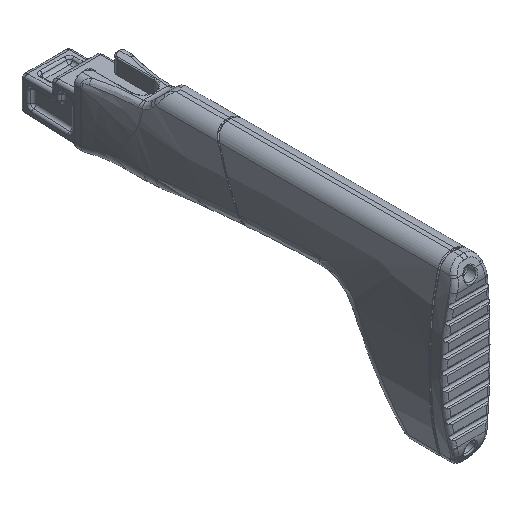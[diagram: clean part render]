
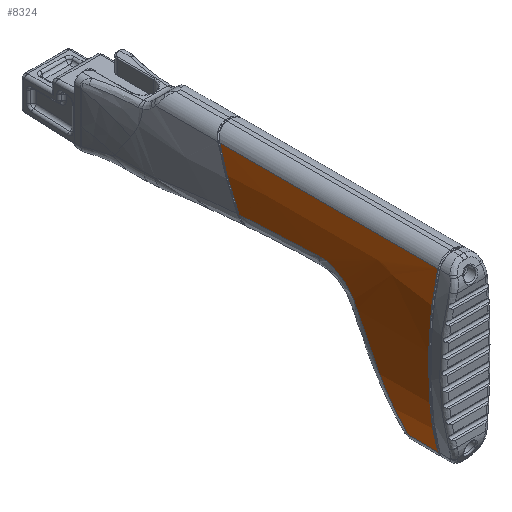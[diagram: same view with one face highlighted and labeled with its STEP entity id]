
A CAD part, isometric view. The second image highlights one B-rep face of the part: STEP entity #8324.
In plain terms, the highlighted free-form (B-spline) face has degree [1, 2] with [2, 5] control points.
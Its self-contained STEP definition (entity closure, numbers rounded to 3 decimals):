
#124=(
BOUNDED_SURFACE()
B_SPLINE_SURFACE(1,2,((#15214,#15215,#15216,#15217,#15218),(#15219,#15220,
#15221,#15222,#15223)),.UNSPECIFIED.,.F.,.F.,.F.)
B_SPLINE_SURFACE_WITH_KNOTS((2,2),(3,2,3),(0.041,2.203),
(-2.476,-1.571,-0.665),.UNSPECIFIED.)
GEOMETRIC_REPRESENTATION_ITEM()
RATIONAL_B_SPLINE_SURFACE(((1.,0.899,1.,0.899,1.),
(1.,0.899,1.,0.899,1.)))
REPRESENTATION_ITEM('')
SURFACE()
);
#330=LINE('',#15212,#699);
#331=LINE('',#15245,#700);
#699=VECTOR('',#9850,10.);
#700=VECTOR('',#9853,10.);
#1283=FACE_OUTER_BOUND('',#1867,.T.);
#1867=EDGE_LOOP('',(#5753,#5754,#5755,#5756,#5757,#5758,#5759,#5760));
#2472=B_SPLINE_CURVE_WITH_KNOTS('',3,(#14835,#14836,#14837,#14838,#14839),
 .UNSPECIFIED.,.F.,.F.,(4,1,4),(1.921,2.158,2.473),
 .UNSPECIFIED.);
#2494=B_SPLINE_CURVE_WITH_KNOTS('',3,(#15196,#15197,#15198,#15199),
 .UNSPECIFIED.,.F.,.F.,(4,4),(-0.016,0.),
 .UNSPECIFIED.);
#2495=B_SPLINE_CURVE_WITH_KNOTS('',3,(#15225,#15226,#15227,#15228),
 .UNSPECIFIED.,.F.,.F.,(4,4),(-10.9,-5.584),
 .UNSPECIFIED.);
#2496=B_SPLINE_CURVE_WITH_KNOTS('',3,(#15230,#15231,#15232,#15233,#15234,
#15235),.UNSPECIFIED.,.F.,.F.,(4,1,1,4),(-3.312,-2.366,
-1.419,0.),.UNSPECIFIED.);
#2497=B_SPLINE_CURVE_WITH_KNOTS('',3,(#15237,#15238,#15239,#15240,#15241,
#15242,#15243),.UNSPECIFIED.,.F.,.F.,(4,1,1,1,4),(-6.528,-5.596,
-4.663,-2.798,0.),.UNSPECIFIED.);
#2498=B_SPLINE_CURVE_WITH_KNOTS('',3,(#15246,#15247,#15248,#15249,#15250,
#15251,#15252,#15253,#15254,#15255,#15256),.UNSPECIFIED.,.F.,.F.,(4,1,1,
1,1,1,1,1,4),(0.,0.763,1.525,3.05,4.575,
7.626,9.151,9.913,10.676),
 .UNSPECIFIED.);
#3386=VERTEX_POINT('',#14824);
#3389=VERTEX_POINT('',#14833);
#3410=VERTEX_POINT('',#15132);
#3417=VERTEX_POINT('',#15211);
#3418=VERTEX_POINT('',#15224);
#3419=VERTEX_POINT('',#15229);
#3420=VERTEX_POINT('',#15236);
#3421=VERTEX_POINT('',#15244);
#4228=EDGE_CURVE('',#3389,#3386,#2472,.T.);
#4266=EDGE_CURVE('',#3410,#3389,#2494,.T.);
#4272=EDGE_CURVE('',#3417,#3386,#330,.T.);
#4274=EDGE_CURVE('',#3418,#3410,#2495,.T.);
#4275=EDGE_CURVE('',#3419,#3418,#2496,.T.);
#4276=EDGE_CURVE('',#3420,#3419,#2497,.T.);
#4277=EDGE_CURVE('',#3420,#3421,#331,.T.);
#4278=EDGE_CURVE('',#3417,#3421,#2498,.T.);
#5753=ORIENTED_EDGE('',*,*,#4228,.F.);
#5754=ORIENTED_EDGE('',*,*,#4266,.F.);
#5755=ORIENTED_EDGE('',*,*,#4274,.F.);
#5756=ORIENTED_EDGE('',*,*,#4275,.F.);
#5757=ORIENTED_EDGE('',*,*,#4276,.F.);
#5758=ORIENTED_EDGE('',*,*,#4277,.T.);
#5759=ORIENTED_EDGE('',*,*,#4278,.F.);
#5760=ORIENTED_EDGE('',*,*,#4272,.T.);
#8324=ADVANCED_FACE('',(#1283),#124,.T.);
#9850=DIRECTION('',(0.,1.,0.));
#9853=DIRECTION('',(0.,-1.,0.));
#14824=CARTESIAN_POINT('',(-10.031,-549.225,133.253));
#14833=CARTESIAN_POINT('',(-15.247,-567.251,103.588));
#14835=CARTESIAN_POINT('Ctrl Pts',(-15.247,-567.251,
103.588));
#14836=CARTESIAN_POINT('Ctrl Pts',(-14.803,-564.228,
108.564));
#14837=CARTESIAN_POINT('Ctrl Pts',(-13.437,-557.479,
119.672));
#14838=CARTESIAN_POINT('Ctrl Pts',(-11.378,-551.886,128.876));
#14839=CARTESIAN_POINT('Ctrl Pts',(-10.031,-549.225,
133.253));
#15132=CARTESIAN_POINT('',(-15.259,-567.335,103.451));
#15196=CARTESIAN_POINT('Ctrl Pts',(-15.259,-567.335,
103.451));
#15197=CARTESIAN_POINT('Ctrl Pts',(-15.255,-567.307,103.497));
#15198=CARTESIAN_POINT('Ctrl Pts',(-15.251,-567.279,
103.542));
#15199=CARTESIAN_POINT('Ctrl Pts',(-15.247,-567.251,
103.588));
#15211=CARTESIAN_POINT('',(-10.031,-694.735,133.253));
#15212=CARTESIAN_POINT('',(-10.031,-697.501,133.253));
#15214=CARTESIAN_POINT('Ctrl Pts',(-10.031,-694.735,133.253));
#15215=CARTESIAN_POINT('Ctrl Pts',(-16.25,-694.735,
113.043));
#15216=CARTESIAN_POINT('Ctrl Pts',(-16.25,-694.735,
80.303));
#15217=CARTESIAN_POINT('Ctrl Pts',(-16.25,-694.735,
47.563));
#15218=CARTESIAN_POINT('Ctrl Pts',(-10.031,-694.735,27.353));
#15219=CARTESIAN_POINT('Ctrl Pts',(-10.031,-549.225,133.253));
#15220=CARTESIAN_POINT('Ctrl Pts',(-16.25,-549.225,
113.043));
#15221=CARTESIAN_POINT('Ctrl Pts',(-16.25,-549.225,
80.303));
#15222=CARTESIAN_POINT('Ctrl Pts',(-16.25,-549.225,
47.563));
#15223=CARTESIAN_POINT('Ctrl Pts',(-10.031,-549.225,27.353));
#15224=CARTESIAN_POINT('',(-15.023,-620.438,105.958));
#15225=CARTESIAN_POINT('Ctrl Pts',(-15.023,-620.438,
105.958));
#15226=CARTESIAN_POINT('Ctrl Pts',(-15.051,-602.718,
105.683));
#15227=CARTESIAN_POINT('Ctrl Pts',(-15.135,-585.006,
104.846));
#15228=CARTESIAN_POINT('Ctrl Pts',(-15.259,-567.335,
103.451));
#15229=CARTESIAN_POINT('',(-16.12,-647.054,88.811));
#15230=CARTESIAN_POINT('Ctrl Pts',(-16.12,-647.054,
88.811));
#15231=CARTESIAN_POINT('Ctrl Pts',(-16.029,-645.699,
91.755));
#15232=CARTESIAN_POINT('Ctrl Pts',(-15.766,-642.052,97.18));
#15233=CARTESIAN_POINT('Ctrl Pts',(-15.225,-633.073,
104.094));
#15234=CARTESIAN_POINT('Ctrl Pts',(-15.016,-625.169,106.031));
#15235=CARTESIAN_POINT('Ctrl Pts',(-15.023,-620.438,
105.958));
#15236=CARTESIAN_POINT('',(-10.031,-674.92,27.353));
#15237=CARTESIAN_POINT('Ctrl Pts',(-10.031,-674.92,27.353));
#15238=CARTESIAN_POINT('Ctrl Pts',(-10.976,-673.632,
30.426));
#15239=CARTESIAN_POINT('Ctrl Pts',(-12.421,-671.02,
36.399));
#15240=CARTESIAN_POINT('Ctrl Pts',(-14.446,-665.738,
48.158));
#15241=CARTESIAN_POINT('Ctrl Pts',(-16.163,-657.746,
65.617));
#15242=CARTESIAN_POINT('Ctrl Pts',(-16.387,-651.061,80.106));
#15243=CARTESIAN_POINT('Ctrl Pts',(-16.12,-647.054,
88.811));
#15244=CARTESIAN_POINT('',(-10.031,-694.735,27.353));
#15245=CARTESIAN_POINT('',(-10.031,-697.501,27.353));
#15246=CARTESIAN_POINT('Ctrl Pts',(-10.031,-694.735,133.253));
#15247=CARTESIAN_POINT('Ctrl Pts',(-10.782,-694.735,
130.811));
#15248=CARTESIAN_POINT('Ctrl Pts',(-12.045,-694.735,
125.859));
#15249=CARTESIAN_POINT('Ctrl Pts',(-13.936,-694.735,
115.844));
#15250=CARTESIAN_POINT('Ctrl Pts',(-15.446,-694.735,
103.181));
#15251=CARTESIAN_POINT('Ctrl Pts',(-16.558,-694.735,82.854));
#15252=CARTESIAN_POINT('Ctrl Pts',(-16.032,-694.735,
62.458));
#15253=CARTESIAN_POINT('Ctrl Pts',(-13.94,-694.735,
44.771));
#15254=CARTESIAN_POINT('Ctrl Pts',(-12.043,-694.735,
34.745));
#15255=CARTESIAN_POINT('Ctrl Pts',(-10.782,-694.735,
29.795));
#15256=CARTESIAN_POINT('Ctrl Pts',(-10.031,-694.735,27.353));
